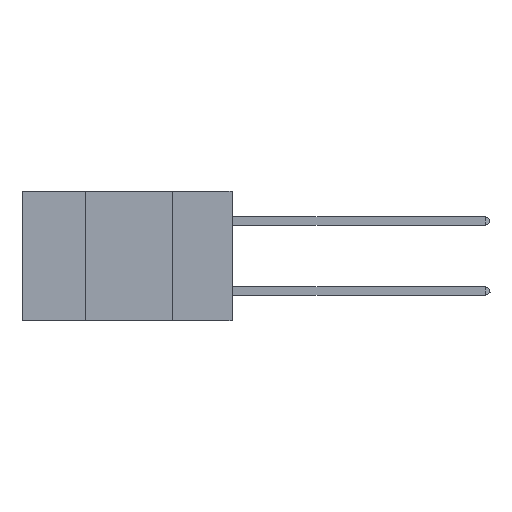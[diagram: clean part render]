
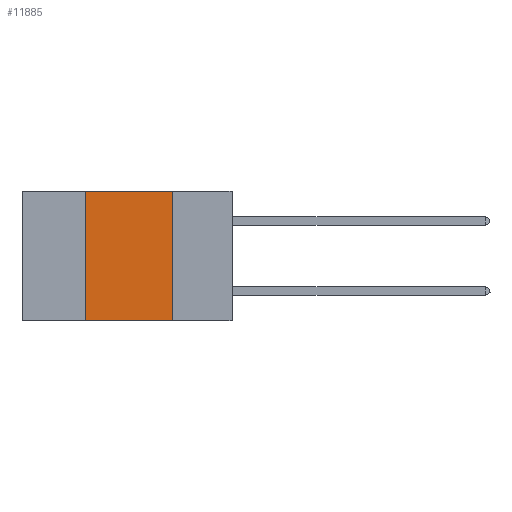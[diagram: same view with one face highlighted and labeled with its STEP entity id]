
A CAD part, left-side view. The second image highlights one B-rep face of the part: STEP entity #11885.
In plain terms, the highlighted planar face has unit normal (-1, 0, 0).
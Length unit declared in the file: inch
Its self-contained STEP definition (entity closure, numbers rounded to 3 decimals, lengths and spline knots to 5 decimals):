
#345 = CARTESIAN_POINT ( 'NONE',  ( 0., 0.17, -0.37 ) ) ;
#821 = LINE ( 'NONE', #8350, #8543 ) ;
#988 = VERTEX_POINT ( 'NONE', #9493 ) ;
#1110 = CARTESIAN_POINT ( 'NONE',  ( 0., 0.17, 0. ) ) ;
#1960 = VERTEX_POINT ( 'NONE', #8154 ) ;
#2142 = CARTESIAN_POINT ( 'NONE',  ( 0., 0.42, 0. ) ) ;
#2476 = CARTESIAN_POINT ( 'NONE',  ( 0., 0.6, -0.37 ) ) ;
#2487 = VERTEX_POINT ( 'NONE', #6984 ) ;
#2558 = EDGE_CURVE ( 'NONE', #2487, #1960, #821, .T. ) ;
#3207 = DIRECTION ( 'NONE',  ( 1., 0., 0. ) ) ;
#3249 = VERTEX_POINT ( 'NONE', #345 ) ;
#3672 = DIRECTION ( 'NONE',  ( 0., 0., -1. ) ) ;
#4093 = EDGE_CURVE ( 'NONE', #988, #2487, #5356, .T. ) ;
#4328 = ORIENTED_EDGE ( 'NONE', *, *, #4093, .F. ) ;
#5356 = LINE ( 'NONE', #2142, #6906 ) ;
#5920 = ORIENTED_EDGE ( 'NONE', *, *, #9427, .F. ) ;
#6906 = VECTOR ( 'NONE', #10954, 39.37008 ) ;
#6984 = CARTESIAN_POINT ( 'NONE',  ( 0., 0.42, 0. ) ) ;
#8154 = CARTESIAN_POINT ( 'NONE',  ( 0., 0.17, 0. ) ) ;
#8350 = CARTESIAN_POINT ( 'NONE',  ( 0., 0.6, 0. ) ) ;
#8543 = VECTOR ( 'NONE', #10723, 39.37008 ) ;
#9337 = EDGE_LOOP ( 'NONE', ( #5920, #12748, #4328, #16017 ) ) ;
#9427 = EDGE_CURVE ( 'NONE', #1960, #3249, #10610, .T. ) ;
#9493 = CARTESIAN_POINT ( 'NONE',  ( 0., 0.42, -0.37 ) ) ;
#10198 = EDGE_CURVE ( 'NONE', #988, #3249, #15632, .T. ) ;
#10574 = PLANE ( 'NONE',  #12194 ) ;
#10610 = LINE ( 'NONE', #1110, #13518 ) ;
#10723 = DIRECTION ( 'NONE',  ( 0., -1., 0. ) ) ;
#10954 = DIRECTION ( 'NONE',  ( 0., 0., 1. ) ) ;
#11885 = ADVANCED_FACE ( 'NONE', ( #12438 ), #10574, .F. ) ;
#12194 = AXIS2_PLACEMENT_3D ( 'NONE', #15677, #3207, #13088 ) ;
#12288 = VECTOR ( 'NONE', #15020, 39.37008 ) ;
#12438 = FACE_OUTER_BOUND ( 'NONE', #9337, .T. ) ;
#12748 = ORIENTED_EDGE ( 'NONE', *, *, #2558, .F. ) ;
#13088 = DIRECTION ( 'NONE',  ( 0., 0., -1. ) ) ;
#13518 = VECTOR ( 'NONE', #3672, 39.37008 ) ;
#15020 = DIRECTION ( 'NONE',  ( 0., -1., 0. ) ) ;
#15632 = LINE ( 'NONE', #2476, #12288 ) ;
#15677 = CARTESIAN_POINT ( 'NONE',  ( 0., 0.6, 0. ) ) ;
#16017 = ORIENTED_EDGE ( 'NONE', *, *, #10198, .T. ) ;
